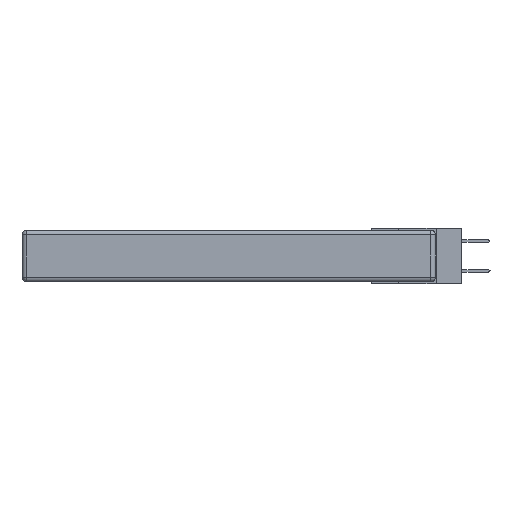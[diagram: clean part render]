
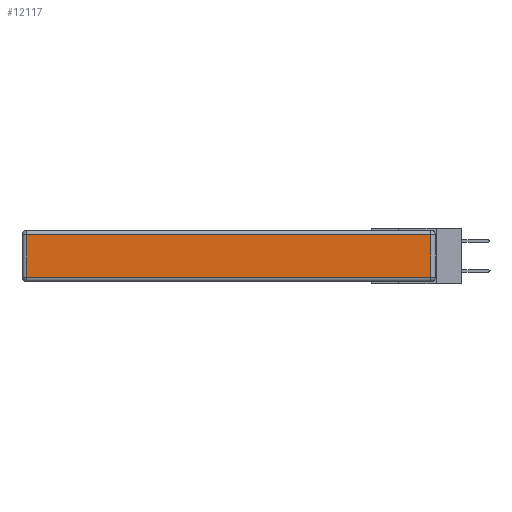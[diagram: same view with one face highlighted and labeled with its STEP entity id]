
A CAD part, left-side view. The second image highlights one B-rep face of the part: STEP entity #12117.
In plain terms, the highlighted planar face has unit normal (-1, 0, 0).
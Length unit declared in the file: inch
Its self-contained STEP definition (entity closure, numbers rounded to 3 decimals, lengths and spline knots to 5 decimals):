
#610 = DIRECTION ( 'NONE',  ( 0., 0., 1. ) ) ;
#754 = ORIENTED_EDGE ( 'NONE', *, *, #17377, .T. ) ;
#878 = LINE ( 'NONE', #9242, #4298 ) ;
#883 = VERTEX_POINT ( 'NONE', #5061 ) ;
#1433 = CARTESIAN_POINT ( 'NONE',  ( 0., 2.75, -0.03 ) ) ;
#2336 = FACE_OUTER_BOUND ( 'NONE', #8241, .T. ) ;
#2353 = VECTOR ( 'NONE', #13568, 39.37008 ) ;
#2587 = VERTEX_POINT ( 'NONE', #14034 ) ;
#4001 = ORIENTED_EDGE ( 'NONE', *, *, #11685, .T. ) ;
#4298 = VECTOR ( 'NONE', #610, 39.37008 ) ;
#4426 = VECTOR ( 'NONE', #18677, 39.37008 ) ;
#4636 = CARTESIAN_POINT ( 'NONE',  ( 0., 0., -0.343 ) ) ;
#5061 = CARTESIAN_POINT ( 'NONE',  ( 0., 0.03, -0.03 ) ) ;
#5873 = VECTOR ( 'NONE', #6084, 39.37008 ) ;
#6084 = DIRECTION ( 'NONE',  ( 0., 0., -1. ) ) ;
#6337 = CARTESIAN_POINT ( 'NONE',  ( 0., 0., -0.313 ) ) ;
#6480 = AXIS2_PLACEMENT_3D ( 'NONE', #4636, #9019, #14759 ) ;
#8085 = VERTEX_POINT ( 'NONE', #18031 ) ;
#8241 = EDGE_LOOP ( 'NONE', ( #4001, #754, #10342, #18637 ) ) ;
#8578 = LINE ( 'NONE', #14380, #5873 ) ;
#9019 = DIRECTION ( 'NONE',  ( -1., 0., 0. ) ) ;
#9242 = CARTESIAN_POINT ( 'NONE',  ( 0., 0.03, -0.343 ) ) ;
#10342 = ORIENTED_EDGE ( 'NONE', *, *, #12379, .T. ) ;
#10747 = CARTESIAN_POINT ( 'NONE',  ( 0., 2.72, -0.03 ) ) ;
#11289 = VERTEX_POINT ( 'NONE', #10747 ) ;
#11685 = EDGE_CURVE ( 'NONE', #8085, #2587, #16639, .T. ) ;
#11828 = PLANE ( 'NONE',  #6480 ) ;
#12117 = ADVANCED_FACE ( 'NONE', ( #2336 ), #11828, .T. ) ;
#12379 = EDGE_CURVE ( 'NONE', #883, #11289, #16194, .T. ) ;
#13568 = DIRECTION ( 'NONE',  ( 0., -1., 0. ) ) ;
#14034 = CARTESIAN_POINT ( 'NONE',  ( 0., 0.03, -0.313 ) ) ;
#14380 = CARTESIAN_POINT ( 'NONE',  ( 0., 2.72, -0.343 ) ) ;
#14759 = DIRECTION ( 'NONE',  ( 0., 0., 1. ) ) ;
#15091 = EDGE_CURVE ( 'NONE', #11289, #8085, #8578, .T. ) ;
#16194 = LINE ( 'NONE', #1433, #4426 ) ;
#16639 = LINE ( 'NONE', #6337, #2353 ) ;
#17377 = EDGE_CURVE ( 'NONE', #2587, #883, #878, .T. ) ;
#18031 = CARTESIAN_POINT ( 'NONE',  ( 0., 2.72, -0.313 ) ) ;
#18637 = ORIENTED_EDGE ( 'NONE', *, *, #15091, .T. ) ;
#18677 = DIRECTION ( 'NONE',  ( 0., 1., 0. ) ) ;
